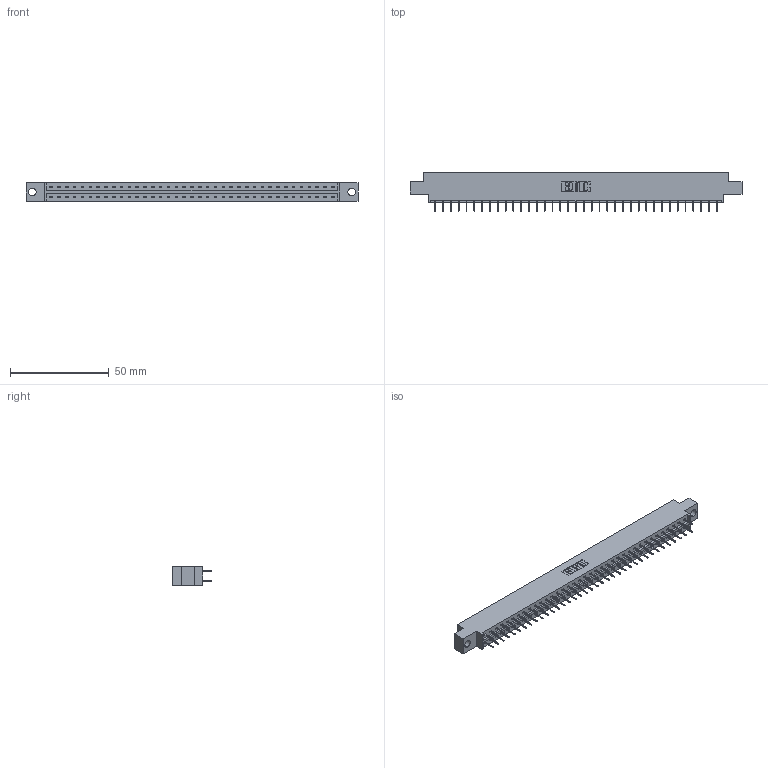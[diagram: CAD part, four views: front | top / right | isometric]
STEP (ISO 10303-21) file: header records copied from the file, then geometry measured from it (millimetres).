
FILE_DESCRIPTION (( 'STEP AP203' ), '1' );
FILE_NAME ('333-074-524-804.STEP', '2018-08-04T21:47:15', ( '' ), ( '' ), 'SwSTEP 2.0', 'SolidWorks 2016', '' );
FILE_SCHEMA (( 'CONFIG_CONTROL_DESIGN' ));
Length unit declared in the file: inch
Products named in the file (3): 333 Part_Offset - .156 Dia - TH; 345-292-001_345-293-124; 333-074-524-804
Assembly tree (75 placements, depth 2):
  333-074-524-804
    333 Part_Offset - .156 Dia - TH
    345-292-001_345-293-124  x74
Bounding box: 168.15 x 19.69 x 9.4 mm (x, y, z)
Volume: 16692.6 mm3; surface area: 19365.2 mm2
Topology: 75 solids, 75 shells, 4262 faces, 12089 edges, 7762 vertices
Faces by surface type: plane 3182, cylinder 1080
Entity records: 24659 total; most frequent: CARTESIAN_POINT 4094, ORIENTED_EDGE 4030, DIRECTION 3507, EDGE_CURVE 2015, VECTOR 1891, LINE 1891, VERTEX_POINT 1338, AXIS2_PLACEMENT_3D 808
